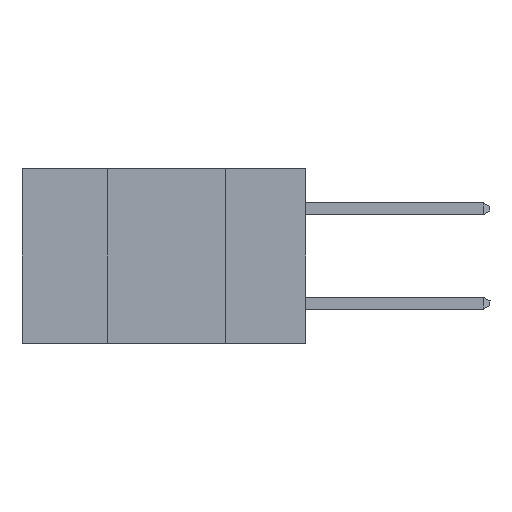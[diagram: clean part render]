
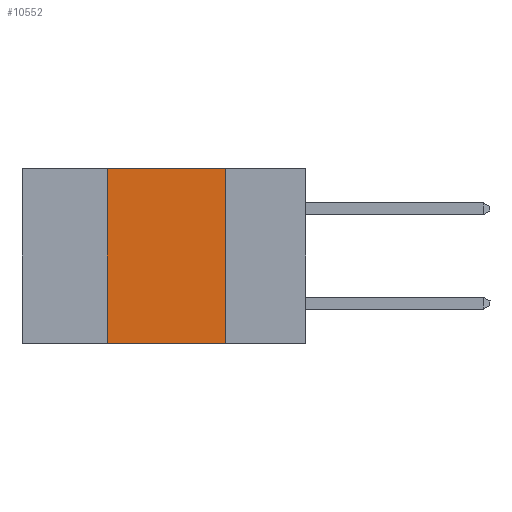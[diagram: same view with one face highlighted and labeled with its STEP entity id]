
A CAD part, left-side view. The second image highlights one B-rep face of the part: STEP entity #10552.
In plain terms, the highlighted planar face has unit normal (-1, 0, 0).
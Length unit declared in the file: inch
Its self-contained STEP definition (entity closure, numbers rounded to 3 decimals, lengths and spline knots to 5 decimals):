
#89 = VERTEX_POINT ( 'NONE', #1712 ) ;
#251 = FACE_OUTER_BOUND ( 'NONE', #6434, .T. ) ;
#1039 = LINE ( 'NONE', #6916, #6773 ) ;
#1154 = CARTESIAN_POINT ( 'NONE',  ( 0., 0.42, 0. ) ) ;
#1251 = CARTESIAN_POINT ( 'NONE',  ( 0., 0.17, 0. ) ) ;
#1429 = DIRECTION ( 'NONE',  ( 0., 0., -1. ) ) ;
#1712 = CARTESIAN_POINT ( 'NONE',  ( 0., 0.17, -0.37 ) ) ;
#1929 = DIRECTION ( 'NONE',  ( 0., -1., 0. ) ) ;
#2228 = VERTEX_POINT ( 'NONE', #1251 ) ;
#2392 = CARTESIAN_POINT ( 'NONE',  ( 0., 0.6, 0. ) ) ;
#2762 = ORIENTED_EDGE ( 'NONE', *, *, #7762, .F. ) ;
#2802 = LINE ( 'NONE', #5551, #7479 ) ;
#2999 = VERTEX_POINT ( 'NONE', #8334 ) ;
#3381 = EDGE_CURVE ( 'NONE', #4841, #2228, #10358, .T. ) ;
#3428 = EDGE_CURVE ( 'NONE', #2228, #89, #2802, .T. ) ;
#3645 = LINE ( 'NONE', #8279, #7516 ) ;
#3887 = VECTOR ( 'NONE', #7330, 39.37008 ) ;
#4841 = VERTEX_POINT ( 'NONE', #1154 ) ;
#5257 = ORIENTED_EDGE ( 'NONE', *, *, #3428, .F. ) ;
#5551 = CARTESIAN_POINT ( 'NONE',  ( 0., 0.17, 0. ) ) ;
#5837 = DIRECTION ( 'NONE',  ( 0., 0., 1. ) ) ;
#6410 = DIRECTION ( 'NONE',  ( 0., 0., -1. ) ) ;
#6434 = EDGE_LOOP ( 'NONE', ( #5257, #7916, #2762, #8417 ) ) ;
#6773 = VECTOR ( 'NONE', #1929, 39.37008 ) ;
#6916 = CARTESIAN_POINT ( 'NONE',  ( 0., 0.6, -0.37 ) ) ;
#7042 = EDGE_CURVE ( 'NONE', #2999, #89, #1039, .T. ) ;
#7071 = AXIS2_PLACEMENT_3D ( 'NONE', #7208, #10573, #1429 ) ;
#7208 = CARTESIAN_POINT ( 'NONE',  ( 0., 0.6, 0. ) ) ;
#7330 = DIRECTION ( 'NONE',  ( 0., -1., 0. ) ) ;
#7479 = VECTOR ( 'NONE', #6410, 39.37008 ) ;
#7516 = VECTOR ( 'NONE', #5837, 39.37008 ) ;
#7762 = EDGE_CURVE ( 'NONE', #2999, #4841, #3645, .T. ) ;
#7916 = ORIENTED_EDGE ( 'NONE', *, *, #3381, .F. ) ;
#8279 = CARTESIAN_POINT ( 'NONE',  ( 0., 0.42, 0. ) ) ;
#8334 = CARTESIAN_POINT ( 'NONE',  ( 0., 0.42, -0.37 ) ) ;
#8417 = ORIENTED_EDGE ( 'NONE', *, *, #7042, .T. ) ;
#10358 = LINE ( 'NONE', #2392, #3887 ) ;
#10552 = ADVANCED_FACE ( 'NONE', ( #251 ), #10680, .F. ) ;
#10573 = DIRECTION ( 'NONE',  ( 1., 0., 0. ) ) ;
#10680 = PLANE ( 'NONE',  #7071 ) ;
